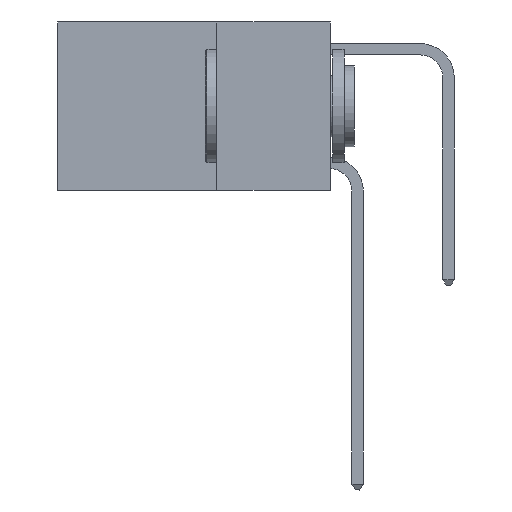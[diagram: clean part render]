
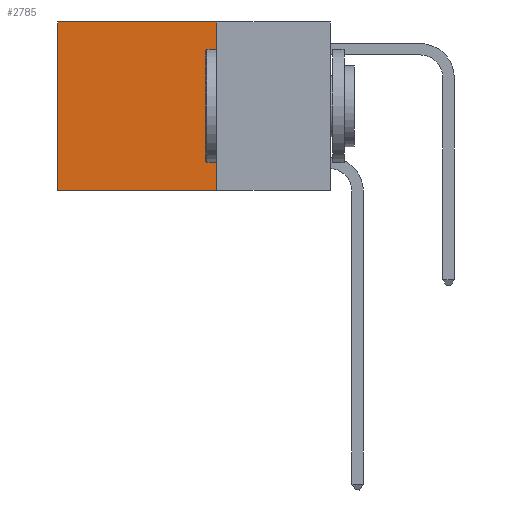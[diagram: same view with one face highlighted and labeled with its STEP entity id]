
A CAD part, left-side view. The second image highlights one B-rep face of the part: STEP entity #2785.
In plain terms, the highlighted planar face has unit normal (-1, 0, 0).
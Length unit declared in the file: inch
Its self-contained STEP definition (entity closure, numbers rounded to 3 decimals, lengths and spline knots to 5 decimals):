
#145 = AXIS2_PLACEMENT_3D ( 'NONE', #16224, #8684, #8498 ) ;
#286 = CARTESIAN_POINT ( 'NONE',  ( 0.2625, 0.25, 0. ) ) ;
#664 = CARTESIAN_POINT ( 'NONE',  ( 0.2625, 0.25, -0.37 ) ) ;
#776 = VECTOR ( 'NONE', #13487, 39.37008 ) ;
#1093 = CARTESIAN_POINT ( 'NONE',  ( 0.2625, 0.6, 0. ) ) ;
#2080 = VERTEX_POINT ( 'NONE', #8188 ) ;
#2298 = DIRECTION ( 'NONE',  ( 0., 0., -1. ) ) ;
#2394 = ORIENTED_EDGE ( 'NONE', *, *, #12357, .T. ) ;
#2785 = ADVANCED_FACE ( 'NONE', ( #5785 ), #3449, .F. ) ;
#3270 = VERTEX_POINT ( 'NONE', #14919 ) ;
#3449 = PLANE ( 'NONE',  #145 ) ;
#4204 = CARTESIAN_POINT ( 'NONE',  ( 0.2625, 0.6, 0. ) ) ;
#4290 = LINE ( 'NONE', #286, #12238 ) ;
#5785 = FACE_OUTER_BOUND ( 'NONE', #7572, .T. ) ;
#7572 = EDGE_LOOP ( 'NONE', ( #14438, #8850, #9594, #2394 ) ) ;
#8187 = CARTESIAN_POINT ( 'NONE',  ( 0.2625, 0.25, -0.37 ) ) ;
#8188 = CARTESIAN_POINT ( 'NONE',  ( 0.2625, 0.25, 0. ) ) ;
#8498 = DIRECTION ( 'NONE',  ( 0., 0., -1. ) ) ;
#8684 = DIRECTION ( 'NONE',  ( 1., 0., 0. ) ) ;
#8850 = ORIENTED_EDGE ( 'NONE', *, *, #9320, .F. ) ;
#8993 = VECTOR ( 'NONE', #11821, 39.37008 ) ;
#9035 = LINE ( 'NONE', #1093, #8993 ) ;
#9320 = EDGE_CURVE ( 'NONE', #9920, #3270, #16145, .T. ) ;
#9594 = ORIENTED_EDGE ( 'NONE', *, *, #13910, .F. ) ;
#9920 = VERTEX_POINT ( 'NONE', #8187 ) ;
#10055 = CARTESIAN_POINT ( 'NONE',  ( 0.2625, 0.25, 0. ) ) ;
#10133 = EDGE_CURVE ( 'NONE', #15125, #3270, #9035, .T. ) ;
#11821 = DIRECTION ( 'NONE',  ( 0., 0., -1. ) ) ;
#12238 = VECTOR ( 'NONE', #14559, 39.37008 ) ;
#12357 = EDGE_CURVE ( 'NONE', #2080, #15125, #4290, .T. ) ;
#12755 = LINE ( 'NONE', #10055, #16079 ) ;
#13487 = DIRECTION ( 'NONE',  ( 0., 1., 0. ) ) ;
#13910 = EDGE_CURVE ( 'NONE', #2080, #9920, #12755, .T. ) ;
#14438 = ORIENTED_EDGE ( 'NONE', *, *, #10133, .T. ) ;
#14559 = DIRECTION ( 'NONE',  ( 0., 1., 0. ) ) ;
#14919 = CARTESIAN_POINT ( 'NONE',  ( 0.2625, 0.6, -0.37 ) ) ;
#15125 = VERTEX_POINT ( 'NONE', #4204 ) ;
#16079 = VECTOR ( 'NONE', #2298, 39.37008 ) ;
#16145 = LINE ( 'NONE', #664, #776 ) ;
#16224 = CARTESIAN_POINT ( 'NONE',  ( 0.2625, 0.25, 0. ) ) ;
